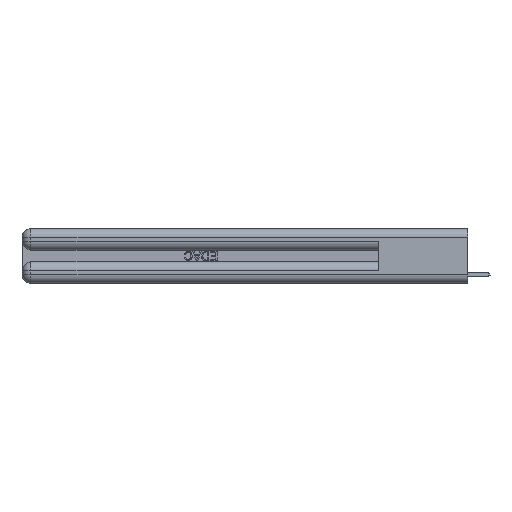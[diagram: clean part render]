
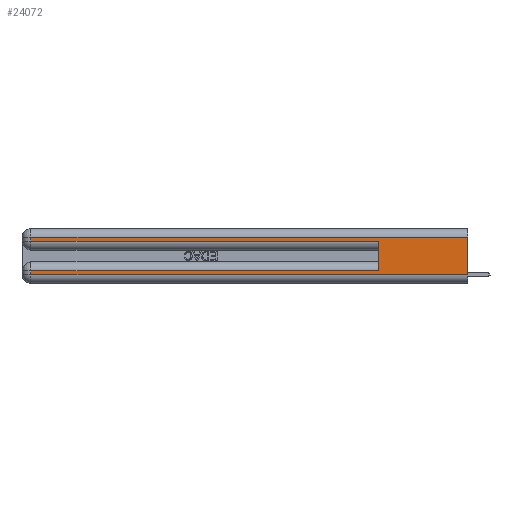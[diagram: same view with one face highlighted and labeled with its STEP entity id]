
A CAD part, left-side view. The second image highlights one B-rep face of the part: STEP entity #24072.
In plain terms, the highlighted planar face has unit normal (-1, 0, 0).
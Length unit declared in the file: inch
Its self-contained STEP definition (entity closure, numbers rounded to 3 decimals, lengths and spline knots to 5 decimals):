
#124 = EDGE_CURVE ( 'NONE', #7390, #10743, #11452, .T. ) ;
#712 = CARTESIAN_POINT ( 'NONE',  ( 0., 0., 0.06 ) ) ;
#1212 = ORIENTED_EDGE ( 'NONE', *, *, #2392, .T. ) ;
#1364 = VERTEX_POINT ( 'NONE', #12933 ) ;
#1450 = VERTEX_POINT ( 'NONE', #26657 ) ;
#1873 = EDGE_LOOP ( 'NONE', ( #26926, #1212, #26545, #21578, #3614, #16387, #19799, #25783 ) ) ;
#1877 = CARTESIAN_POINT ( 'NONE',  ( 0., 0.6, 0.285 ) ) ;
#2127 = VECTOR ( 'NONE', #19599, 39.37008 ) ;
#2392 = EDGE_CURVE ( 'NONE', #26641, #1364, #21093, .T. ) ;
#2678 = VECTOR ( 'NONE', #25781, 39.37008 ) ;
#3438 = LINE ( 'NONE', #712, #18066 ) ;
#3614 = ORIENTED_EDGE ( 'NONE', *, *, #17775, .F. ) ;
#3847 = VECTOR ( 'NONE', #20796, 39.37008 ) ;
#4368 = LINE ( 'NONE', #26415, #17133 ) ;
#4575 = CARTESIAN_POINT ( 'NONE',  ( 0., 0., 0.06 ) ) ;
#5758 = FACE_OUTER_BOUND ( 'NONE', #1873, .T. ) ;
#6249 = DIRECTION ( 'NONE',  ( 0., 0., -1. ) ) ;
#6949 = CARTESIAN_POINT ( 'NONE',  ( 0., 0., 0.285 ) ) ;
#7201 = EDGE_CURVE ( 'NONE', #1450, #16189, #13657, .T. ) ;
#7345 = CARTESIAN_POINT ( 'NONE',  ( 0., 0.6, 0.145 ) ) ;
#7390 = VERTEX_POINT ( 'NONE', #26352 ) ;
#7982 = CARTESIAN_POINT ( 'NONE',  ( 0., 0., 0.37 ) ) ;
#9301 = EDGE_CURVE ( 'NONE', #16189, #16131, #3438, .T. ) ;
#10687 = CARTESIAN_POINT ( 'NONE',  ( 0., 2.94, 0.37 ) ) ;
#10743 = VERTEX_POINT ( 'NONE', #1877 ) ;
#11133 = EDGE_CURVE ( 'NONE', #1364, #7390, #13019, .T. ) ;
#11452 = LINE ( 'NONE', #6949, #3847 ) ;
#11460 = CARTESIAN_POINT ( 'NONE',  ( 0., 2.94, 0.37 ) ) ;
#12031 = DIRECTION ( 'NONE',  ( 1., 0., 0. ) ) ;
#12320 = DIRECTION ( 'NONE',  ( 0., -1., 0. ) ) ;
#12933 = CARTESIAN_POINT ( 'NONE',  ( 0., 2.94, 0.31 ) ) ;
#13019 = LINE ( 'NONE', #10687, #2127 ) ;
#13473 = EDGE_CURVE ( 'NONE', #20280, #1450, #16093, .T. ) ;
#13657 = LINE ( 'NONE', #11460, #25867 ) ;
#14498 = CARTESIAN_POINT ( 'NONE',  ( 0., 0., 0.085 ) ) ;
#16093 = LINE ( 'NONE', #14498, #17773 ) ;
#16131 = VERTEX_POINT ( 'NONE', #4575 ) ;
#16189 = VERTEX_POINT ( 'NONE', #25430 ) ;
#16387 = ORIENTED_EDGE ( 'NONE', *, *, #13473, .T. ) ;
#17133 = VECTOR ( 'NONE', #6249, 39.37008 ) ;
#17773 = VECTOR ( 'NONE', #23396, 39.37008 ) ;
#17775 = EDGE_CURVE ( 'NONE', #20280, #10743, #27358, .T. ) ;
#18066 = VECTOR ( 'NONE', #12320, 39.37008 ) ;
#19505 = AXIS2_PLACEMENT_3D ( 'NONE', #7982, #12031, #27973 ) ;
#19599 = DIRECTION ( 'NONE',  ( 0., 0., -1. ) ) ;
#19799 = ORIENTED_EDGE ( 'NONE', *, *, #7201, .T. ) ;
#20169 = VECTOR ( 'NONE', #26422, 39.37008 ) ;
#20223 = CARTESIAN_POINT ( 'NONE',  ( 0., 0.6, 0.085 ) ) ;
#20280 = VERTEX_POINT ( 'NONE', #20223 ) ;
#20382 = DIRECTION ( 'NONE',  ( 0., 0., -1. ) ) ;
#20796 = DIRECTION ( 'NONE',  ( 0., -1., 0. ) ) ;
#21093 = LINE ( 'NONE', #25650, #2678 ) ;
#21578 = ORIENTED_EDGE ( 'NONE', *, *, #124, .T. ) ;
#23001 = CARTESIAN_POINT ( 'NONE',  ( 0., 0., 0.31 ) ) ;
#23396 = DIRECTION ( 'NONE',  ( 0., 1., 0. ) ) ;
#23466 = EDGE_CURVE ( 'NONE', #26641, #16131, #4368, .T. ) ;
#24072 = ADVANCED_FACE ( 'NONE', ( #5758 ), #25634, .F. ) ;
#25430 = CARTESIAN_POINT ( 'NONE',  ( 0., 2.94, 0.06 ) ) ;
#25634 = PLANE ( 'NONE',  #19505 ) ;
#25650 = CARTESIAN_POINT ( 'NONE',  ( 0., 0., 0.31 ) ) ;
#25781 = DIRECTION ( 'NONE',  ( 0., 1., 0. ) ) ;
#25783 = ORIENTED_EDGE ( 'NONE', *, *, #9301, .T. ) ;
#25867 = VECTOR ( 'NONE', #20382, 39.37008 ) ;
#26352 = CARTESIAN_POINT ( 'NONE',  ( 0., 2.94, 0.285 ) ) ;
#26415 = CARTESIAN_POINT ( 'NONE',  ( 0., 0., 0.37 ) ) ;
#26422 = DIRECTION ( 'NONE',  ( 0., 0., 1. ) ) ;
#26545 = ORIENTED_EDGE ( 'NONE', *, *, #11133, .T. ) ;
#26641 = VERTEX_POINT ( 'NONE', #23001 ) ;
#26657 = CARTESIAN_POINT ( 'NONE',  ( 0., 2.94, 0.085 ) ) ;
#26926 = ORIENTED_EDGE ( 'NONE', *, *, #23466, .F. ) ;
#27358 = LINE ( 'NONE', #7345, #20169 ) ;
#27973 = DIRECTION ( 'NONE',  ( 0., 0., -1. ) ) ;
